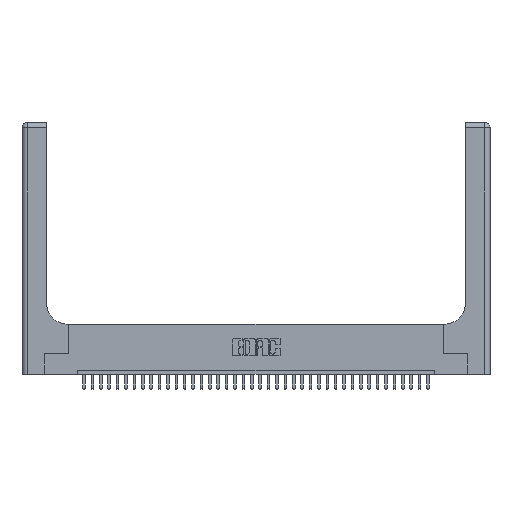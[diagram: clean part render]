
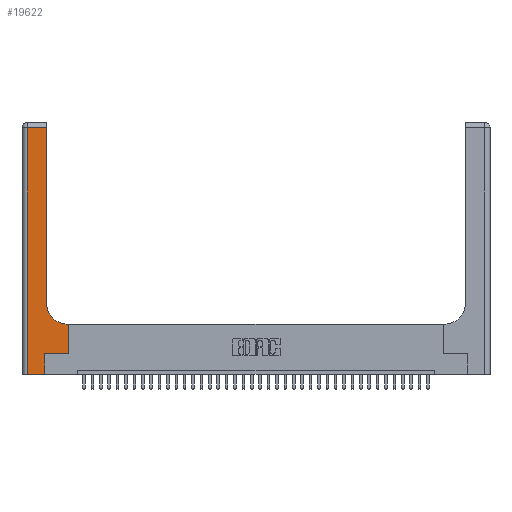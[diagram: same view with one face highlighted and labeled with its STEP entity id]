
A CAD part, top view. The second image highlights one B-rep face of the part: STEP entity #19622.
In plain terms, the highlighted planar face has unit normal (0, 0, 1).
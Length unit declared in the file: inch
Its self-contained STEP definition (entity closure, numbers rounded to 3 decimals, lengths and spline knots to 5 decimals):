
#243 = VECTOR ( 'NONE', #14718, 39.37008 ) ;
#1378 = VECTOR ( 'NONE', #29775, 39.37008 ) ;
#2040 = ORIENTED_EDGE ( 'NONE', *, *, #11856, .T. ) ;
#3269 = VERTEX_POINT ( 'NONE', #14562 ) ;
#3275 = CARTESIAN_POINT ( 'NONE',  ( 0.269, 0.25, 0.37 ) ) ;
#3462 = EDGE_CURVE ( 'NONE', #28096, #19125, #24944, .T. ) ;
#4295 = CARTESIAN_POINT ( 'NONE',  ( 0.5585, 0.25, 0.37 ) ) ;
#4429 = EDGE_CURVE ( 'NONE', #9450, #34314, #21770, .T. ) ;
#5204 = FACE_OUTER_BOUND ( 'NONE', #15301, .T. ) ;
#5360 = ORIENTED_EDGE ( 'NONE', *, *, #26986, .T. ) ;
#5679 = CARTESIAN_POINT ( 'NONE',  ( 0.2915, 0.85, 0.37 ) ) ;
#5771 = LINE ( 'NONE', #7820, #35238 ) ;
#5804 = EDGE_CURVE ( 'NONE', #3269, #28096, #23000, .T. ) ;
#5966 = DIRECTION ( 'NONE',  ( 1., 0., 0. ) ) ;
#6119 = VECTOR ( 'NONE', #15772, 39.37008 ) ;
#6277 = DIRECTION ( 'NONE',  ( -1., 0., 0. ) ) ;
#6671 = CARTESIAN_POINT ( 'NONE',  ( 0.06, 0., 0.37 ) ) ;
#7820 = CARTESIAN_POINT ( 'NONE',  ( 0.269, 0., 0.37 ) ) ;
#8373 = DIRECTION ( 'NONE',  ( 0., -1., 0. ) ) ;
#8693 = ORIENTED_EDGE ( 'NONE', *, *, #33497, .T. ) ;
#9272 = CARTESIAN_POINT ( 'NONE',  ( 0.5585, 0.25, 0.37 ) ) ;
#9450 = VERTEX_POINT ( 'NONE', #34839 ) ;
#10721 = ORIENTED_EDGE ( 'NONE', *, *, #12860, .T. ) ;
#11076 = EDGE_CURVE ( 'NONE', #19125, #31537, #26731, .T. ) ;
#11618 = VERTEX_POINT ( 'NONE', #5679 ) ;
#11856 = EDGE_CURVE ( 'NONE', #31167, #9450, #17711, .T. ) ;
#11989 = DIRECTION ( 'NONE',  ( 0., 0., -1. ) ) ;
#12860 = EDGE_CURVE ( 'NONE', #11618, #3269, #30323, .T. ) ;
#14562 = CARTESIAN_POINT ( 'NONE',  ( 0.2915, 2.94, 0.37 ) ) ;
#14718 = DIRECTION ( 'NONE',  ( 1., 0., 0. ) ) ;
#15301 = EDGE_LOOP ( 'NONE', ( #10721, #32285, #23932, #15530, #8693, #5360, #2040, #30497, #17721 ) ) ;
#15530 = ORIENTED_EDGE ( 'NONE', *, *, #11076, .T. ) ;
#15687 = CARTESIAN_POINT ( 'NONE',  ( 0.2915, 3., 0.37 ) ) ;
#15772 = DIRECTION ( 'NONE',  ( 0., 1., 0. ) ) ;
#15853 = CARTESIAN_POINT ( 'NONE',  ( 0.06, 3., 0.37 ) ) ;
#16641 = AXIS2_PLACEMENT_3D ( 'NONE', #34273, #23056, #20269 ) ;
#16822 = DIRECTION ( 'NONE',  ( 0., 1., 0. ) ) ;
#17500 = CARTESIAN_POINT ( 'NONE',  ( 0.2915, 0.6, 0.37 ) ) ;
#17711 = LINE ( 'NONE', #4295, #6119 ) ;
#17721 = ORIENTED_EDGE ( 'NONE', *, *, #28201, .T. ) ;
#17746 = VECTOR ( 'NONE', #8373, 39.37008 ) ;
#17977 = DIRECTION ( 'NONE',  ( -1., 0., 0. ) ) ;
#18090 = VECTOR ( 'NONE', #24283, 39.37008 ) ;
#18595 = AXIS2_PLACEMENT_3D ( 'NONE', #26208, #11989, #17977 ) ;
#19125 = VERTEX_POINT ( 'NONE', #6671 ) ;
#19419 = CARTESIAN_POINT ( 'NONE',  ( 0.06, 2.94, 0.37 ) ) ;
#19622 = ADVANCED_FACE ( 'NONE', ( #5204 ), #26087, .F. ) ;
#20269 = DIRECTION ( 'NONE',  ( 1., 0., 0. ) ) ;
#21770 = LINE ( 'NONE', #17500, #31574 ) ;
#22038 = LINE ( 'NONE', #3275, #243 ) ;
#23000 = LINE ( 'NONE', #24643, #18090 ) ;
#23056 = DIRECTION ( 'NONE',  ( 0., 0., -1. ) ) ;
#23932 = ORIENTED_EDGE ( 'NONE', *, *, #3462, .T. ) ;
#24283 = DIRECTION ( 'NONE',  ( -1., 0., 0. ) ) ;
#24484 = VECTOR ( 'NONE', #5966, 39.37008 ) ;
#24643 = CARTESIAN_POINT ( 'NONE',  ( 0., 2.94, 0.37 ) ) ;
#24944 = LINE ( 'NONE', #15853, #17746 ) ;
#25858 = CARTESIAN_POINT ( 'NONE',  ( 0.5415, 0.6, 0.37 ) ) ;
#26087 = PLANE ( 'NONE',  #18595 ) ;
#26208 = CARTESIAN_POINT ( 'NONE',  ( 0., 3., 0.37 ) ) ;
#26731 = LINE ( 'NONE', #28793, #24484 ) ;
#26823 = CIRCLE ( 'NONE', #16641, 0.25 ) ;
#26986 = EDGE_CURVE ( 'NONE', #35770, #31167, #22038, .T. ) ;
#28096 = VERTEX_POINT ( 'NONE', #19419 ) ;
#28201 = EDGE_CURVE ( 'NONE', #34314, #11618, #26823, .T. ) ;
#28793 = CARTESIAN_POINT ( 'NONE',  ( 0., 0., 0.37 ) ) ;
#29775 = DIRECTION ( 'NONE',  ( 0., 1., 0. ) ) ;
#30031 = CARTESIAN_POINT ( 'NONE',  ( 0.269, 0.25, 0.37 ) ) ;
#30323 = LINE ( 'NONE', #15687, #1378 ) ;
#30497 = ORIENTED_EDGE ( 'NONE', *, *, #4429, .T. ) ;
#31167 = VERTEX_POINT ( 'NONE', #9272 ) ;
#31537 = VERTEX_POINT ( 'NONE', #33968 ) ;
#31574 = VECTOR ( 'NONE', #6277, 39.37008 ) ;
#32285 = ORIENTED_EDGE ( 'NONE', *, *, #5804, .T. ) ;
#33497 = EDGE_CURVE ( 'NONE', #31537, #35770, #5771, .T. ) ;
#33968 = CARTESIAN_POINT ( 'NONE',  ( 0.269, 0., 0.37 ) ) ;
#34273 = CARTESIAN_POINT ( 'NONE',  ( 0.5415, 0.85, 0.37 ) ) ;
#34314 = VERTEX_POINT ( 'NONE', #25858 ) ;
#34839 = CARTESIAN_POINT ( 'NONE',  ( 0.5585, 0.6, 0.37 ) ) ;
#35238 = VECTOR ( 'NONE', #16822, 39.37008 ) ;
#35770 = VERTEX_POINT ( 'NONE', #30031 ) ;
